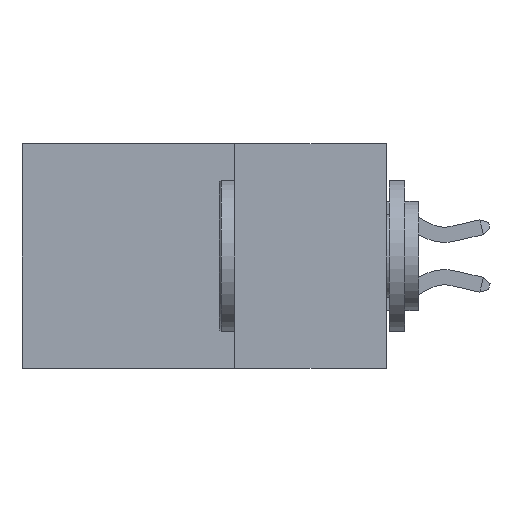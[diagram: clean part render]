
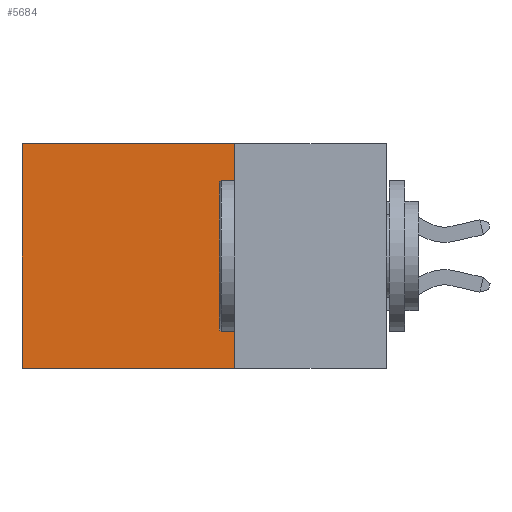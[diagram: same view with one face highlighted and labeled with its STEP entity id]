
A CAD part, left-side view. The second image highlights one B-rep face of the part: STEP entity #5684.
In plain terms, the highlighted planar face has unit normal (-1, 0, 0).
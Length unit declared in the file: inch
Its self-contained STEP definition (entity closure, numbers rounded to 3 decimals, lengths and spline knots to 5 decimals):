
#339 = LINE ( 'NONE', #3642, #10476 ) ;
#1559 = DIRECTION ( 'NONE',  ( 0., 0., -1. ) ) ;
#2357 = DIRECTION ( 'NONE',  ( 1., 0., 0. ) ) ;
#3048 = VERTEX_POINT ( 'NONE', #17940 ) ;
#3062 = CARTESIAN_POINT ( 'NONE',  ( 0.2615, 0.25, -0.37 ) ) ;
#3597 = EDGE_CURVE ( 'NONE', #3048, #20127, #7278, .T. ) ;
#3642 = CARTESIAN_POINT ( 'NONE',  ( 0.2615, 0.6, -0.37 ) ) ;
#3727 = VERTEX_POINT ( 'NONE', #7125 ) ;
#3899 = ORIENTED_EDGE ( 'NONE', *, *, #11907, .T. ) ;
#4274 = PLANE ( 'NONE',  #11312 ) ;
#4402 = ORIENTED_EDGE ( 'NONE', *, *, #3597, .F. ) ;
#5684 = ADVANCED_FACE ( 'NONE', ( #8447 ), #4274, .F. ) ;
#6678 = VECTOR ( 'NONE', #14252, 39.37008 ) ;
#7125 = CARTESIAN_POINT ( 'NONE',  ( 0.2615, 0.6, -0.37 ) ) ;
#7278 = LINE ( 'NONE', #15380, #6678 ) ;
#8249 = EDGE_LOOP ( 'NONE', ( #3899, #18428, #4402, #24121 ) ) ;
#8447 = FACE_OUTER_BOUND ( 'NONE', #8249, .T. ) ;
#10476 = VECTOR ( 'NONE', #14884, 39.37008 ) ;
#11312 = AXIS2_PLACEMENT_3D ( 'NONE', #3062, #2357, #1559 ) ;
#11907 = EDGE_CURVE ( 'NONE', #16134, #3727, #339, .T. ) ;
#12473 = DIRECTION ( 'NONE',  ( 0., 1., 0. ) ) ;
#12572 = VECTOR ( 'NONE', #21464, 39.37008 ) ;
#14252 = DIRECTION ( 'NONE',  ( 0., 0., -1. ) ) ;
#14768 = EDGE_CURVE ( 'NONE', #20127, #3727, #22235, .T. ) ;
#14884 = DIRECTION ( 'NONE',  ( 0., 0., -1. ) ) ;
#15380 = CARTESIAN_POINT ( 'NONE',  ( 0.2615, 0.25, -0.37 ) ) ;
#16134 = VERTEX_POINT ( 'NONE', #22611 ) ;
#16401 = EDGE_CURVE ( 'NONE', #3048, #16134, #21284, .T. ) ;
#17727 = CARTESIAN_POINT ( 'NONE',  ( 0.2615, 0.25, 0. ) ) ;
#17940 = CARTESIAN_POINT ( 'NONE',  ( 0.2615, 0.25, 0. ) ) ;
#17996 = CARTESIAN_POINT ( 'NONE',  ( 0.2615, 0.25, -0.37 ) ) ;
#18428 = ORIENTED_EDGE ( 'NONE', *, *, #14768, .F. ) ;
#20127 = VERTEX_POINT ( 'NONE', #20393 ) ;
#20393 = CARTESIAN_POINT ( 'NONE',  ( 0.2615, 0.25, -0.37 ) ) ;
#21284 = LINE ( 'NONE', #17727, #12572 ) ;
#21464 = DIRECTION ( 'NONE',  ( 0., 1., 0. ) ) ;
#22235 = LINE ( 'NONE', #17996, #22832 ) ;
#22611 = CARTESIAN_POINT ( 'NONE',  ( 0.2615, 0.6, 0. ) ) ;
#22832 = VECTOR ( 'NONE', #12473, 39.37008 ) ;
#24121 = ORIENTED_EDGE ( 'NONE', *, *, #16401, .T. ) ;
